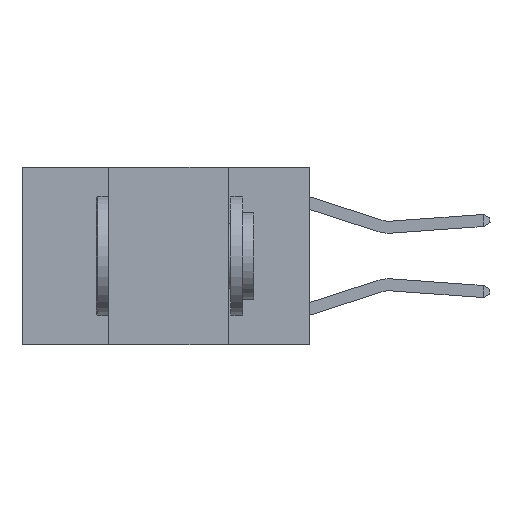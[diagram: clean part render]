
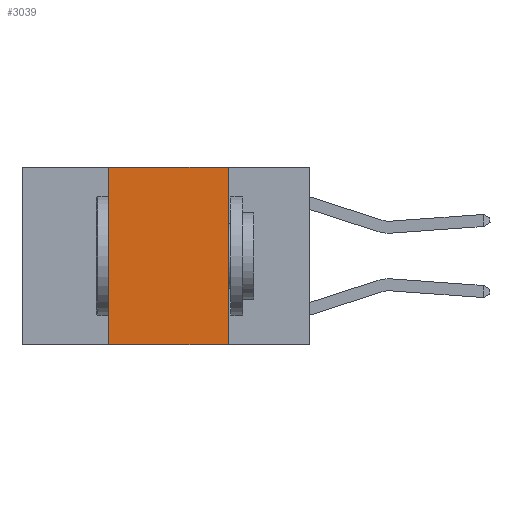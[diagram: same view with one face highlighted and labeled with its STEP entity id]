
A CAD part, left-side view. The second image highlights one B-rep face of the part: STEP entity #3039.
In plain terms, the highlighted planar face has unit normal (-1, 0, 0).
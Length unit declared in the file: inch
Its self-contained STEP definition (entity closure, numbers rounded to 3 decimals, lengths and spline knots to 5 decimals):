
#62 = LINE ( 'NONE', #15307, #10937 ) ;
#104 = EDGE_CURVE ( 'NONE', #10422, #14835, #4146, .T. ) ;
#147 = CARTESIAN_POINT ( 'NONE',  ( 0., 0.6, -0.37 ) ) ;
#252 = EDGE_CURVE ( 'NONE', #10422, #7004, #62, .T. ) ;
#869 = CARTESIAN_POINT ( 'NONE',  ( 0., 0.42, -0.37 ) ) ;
#1025 = CARTESIAN_POINT ( 'NONE',  ( 0., 0.42, 0. ) ) ;
#1183 = ORIENTED_EDGE ( 'NONE', *, *, #4630, .F. ) ;
#2188 = CARTESIAN_POINT ( 'NONE',  ( 0., 0.17, 0. ) ) ;
#2323 = VECTOR ( 'NONE', #12422, 39.37008 ) ;
#3039 = ADVANCED_FACE ( 'NONE', ( #11274 ), #3091, .F. ) ;
#3091 = PLANE ( 'NONE',  #7649 ) ;
#4036 = EDGE_CURVE ( 'NONE', #13498, #14835, #13106, .T. ) ;
#4146 = LINE ( 'NONE', #147, #2323 ) ;
#4630 = EDGE_CURVE ( 'NONE', #7004, #13498, #10684, .T. ) ;
#5052 = CARTESIAN_POINT ( 'NONE',  ( 0., 0.6, 0. ) ) ;
#5497 = DIRECTION ( 'NONE',  ( 0., 0., 1. ) ) ;
#5755 = VECTOR ( 'NONE', #14847, 39.37008 ) ;
#6815 = CARTESIAN_POINT ( 'NONE',  ( 0., 0.17, -0.37 ) ) ;
#7004 = VERTEX_POINT ( 'NONE', #1025 ) ;
#7557 = ORIENTED_EDGE ( 'NONE', *, *, #104, .T. ) ;
#7649 = AXIS2_PLACEMENT_3D ( 'NONE', #16768, #8567, #14076 ) ;
#7696 = DIRECTION ( 'NONE',  ( 0., 0., -1. ) ) ;
#8567 = DIRECTION ( 'NONE',  ( 1., 0., 0. ) ) ;
#10422 = VERTEX_POINT ( 'NONE', #869 ) ;
#10684 = LINE ( 'NONE', #5052, #5755 ) ;
#10937 = VECTOR ( 'NONE', #5497, 39.37008 ) ;
#11274 = FACE_OUTER_BOUND ( 'NONE', #13794, .T. ) ;
#12422 = DIRECTION ( 'NONE',  ( 0., -1., 0. ) ) ;
#12813 = CARTESIAN_POINT ( 'NONE',  ( 0., 0.17, 0. ) ) ;
#13106 = LINE ( 'NONE', #2188, #14541 ) ;
#13498 = VERTEX_POINT ( 'NONE', #12813 ) ;
#13794 = EDGE_LOOP ( 'NONE', ( #16150, #1183, #17388, #7557 ) ) ;
#14076 = DIRECTION ( 'NONE',  ( 0., 0., -1. ) ) ;
#14541 = VECTOR ( 'NONE', #7696, 39.37008 ) ;
#14835 = VERTEX_POINT ( 'NONE', #6815 ) ;
#14847 = DIRECTION ( 'NONE',  ( 0., -1., 0. ) ) ;
#15307 = CARTESIAN_POINT ( 'NONE',  ( 0., 0.42, 0. ) ) ;
#16150 = ORIENTED_EDGE ( 'NONE', *, *, #4036, .F. ) ;
#16768 = CARTESIAN_POINT ( 'NONE',  ( 0., 0.6, 0. ) ) ;
#17388 = ORIENTED_EDGE ( 'NONE', *, *, #252, .F. ) ;
